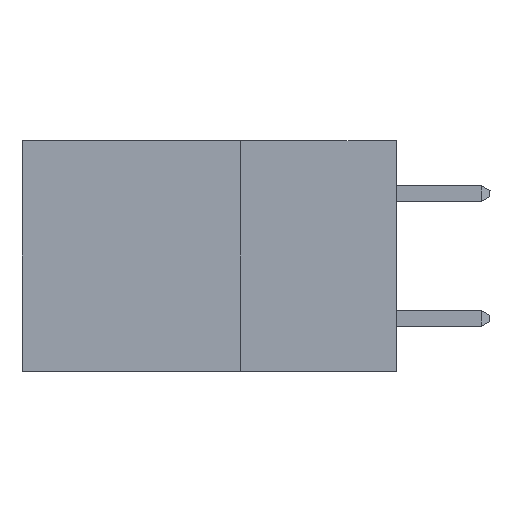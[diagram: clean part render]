
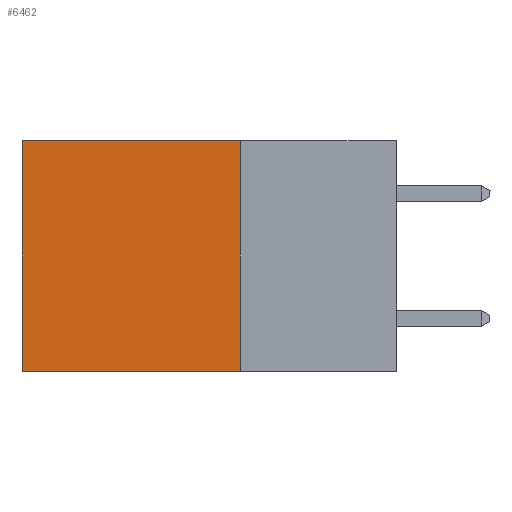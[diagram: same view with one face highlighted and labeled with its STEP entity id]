
A CAD part, left-side view. The second image highlights one B-rep face of the part: STEP entity #6462.
In plain terms, the highlighted planar face has unit normal (-1, 0, 0).
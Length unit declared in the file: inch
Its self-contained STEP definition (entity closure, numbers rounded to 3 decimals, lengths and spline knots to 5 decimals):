
#226 = CARTESIAN_POINT ( 'NONE',  ( 0.298, 0.6, -0.37 ) ) ;
#471 = ORIENTED_EDGE ( 'NONE', *, *, #3581, .F. ) ;
#798 = LINE ( 'NONE', #11339, #14256 ) ;
#845 = VERTEX_POINT ( 'NONE', #1470 ) ;
#1313 = VECTOR ( 'NONE', #10809, 39.37008 ) ;
#1351 = CARTESIAN_POINT ( 'NONE',  ( 0.298, 0.6, 0. ) ) ;
#1470 = CARTESIAN_POINT ( 'NONE',  ( 0.298, 0.25, 0. ) ) ;
#1474 = ORIENTED_EDGE ( 'NONE', *, *, #5566, .T. ) ;
#1644 = CARTESIAN_POINT ( 'NONE',  ( 0.298, 0.25, -0.37 ) ) ;
#1915 = VERTEX_POINT ( 'NONE', #1644 ) ;
#3581 = EDGE_CURVE ( 'NONE', #1915, #16252, #798, .T. ) ;
#3651 = DIRECTION ( 'NONE',  ( 0., 1., 0. ) ) ;
#3887 = VECTOR ( 'NONE', #6205, 39.37008 ) ;
#4096 = ORIENTED_EDGE ( 'NONE', *, *, #8140, .T. ) ;
#4927 = CARTESIAN_POINT ( 'NONE',  ( 0.298, 0.25, 0. ) ) ;
#5064 = LINE ( 'NONE', #9525, #1313 ) ;
#5162 = VECTOR ( 'NONE', #7342, 39.37008 ) ;
#5550 = DIRECTION ( 'NONE',  ( 1., 0., 0. ) ) ;
#5566 = EDGE_CURVE ( 'NONE', #845, #6932, #14017, .T. ) ;
#6205 = DIRECTION ( 'NONE',  ( 0., 1., 0. ) ) ;
#6283 = ORIENTED_EDGE ( 'NONE', *, *, #11931, .F. ) ;
#6462 = ADVANCED_FACE ( 'NONE', ( #7637 ), #14305, .F. ) ;
#6932 = VERTEX_POINT ( 'NONE', #1351 ) ;
#7342 = DIRECTION ( 'NONE',  ( 0., 0., -1. ) ) ;
#7637 = FACE_OUTER_BOUND ( 'NONE', #10326, .T. ) ;
#8140 = EDGE_CURVE ( 'NONE', #6932, #16252, #11190, .T. ) ;
#9525 = CARTESIAN_POINT ( 'NONE',  ( 0.298, 0.25, 0. ) ) ;
#10326 = EDGE_LOOP ( 'NONE', ( #4096, #471, #6283, #1474 ) ) ;
#10668 = CARTESIAN_POINT ( 'NONE',  ( 0.298, 0.25, 0. ) ) ;
#10809 = DIRECTION ( 'NONE',  ( 0., 0., -1. ) ) ;
#11190 = LINE ( 'NONE', #14905, #5162 ) ;
#11339 = CARTESIAN_POINT ( 'NONE',  ( 0.298, 0.25, -0.37 ) ) ;
#11931 = EDGE_CURVE ( 'NONE', #845, #1915, #5064, .T. ) ;
#13903 = AXIS2_PLACEMENT_3D ( 'NONE', #10668, #5550, #14418 ) ;
#14017 = LINE ( 'NONE', #4927, #3887 ) ;
#14256 = VECTOR ( 'NONE', #3651, 39.37008 ) ;
#14305 = PLANE ( 'NONE',  #13903 ) ;
#14418 = DIRECTION ( 'NONE',  ( 0., 0., -1. ) ) ;
#14905 = CARTESIAN_POINT ( 'NONE',  ( 0.298, 0.6, 0. ) ) ;
#16252 = VERTEX_POINT ( 'NONE', #226 ) ;
